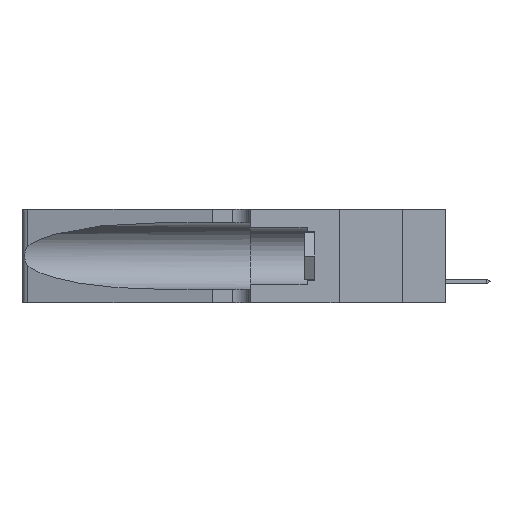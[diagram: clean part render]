
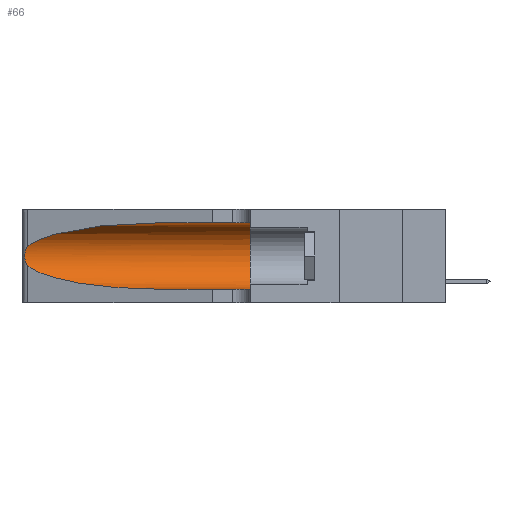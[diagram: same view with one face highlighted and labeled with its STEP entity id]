
A CAD part, left-side view. The second image highlights one B-rep face of the part: STEP entity #66.
In plain terms, the highlighted cylindrical face has radius 3.308 mm (diameter 6.617 mm), a partial arc.
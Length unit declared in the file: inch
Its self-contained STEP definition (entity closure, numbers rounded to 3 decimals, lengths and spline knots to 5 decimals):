
#31 = CARTESIAN_POINT ( 'NONE',  ( 0.25555, 1.22994, 0.2215 ) ) ;
#66 = ADVANCED_FACE ( 'NONE', ( #11929 ), #21941, .F. ) ;
#129 = CARTESIAN_POINT ( 'NONE',  ( 0.2373, 1.15595, 0.28018 ) ) ;
#564 = CARTESIAN_POINT ( 'NONE',  ( 0.1305, 1.61858, 0.185 ) ) ;
#613 = ORIENTED_EDGE ( 'NONE', *, *, #24819, .T. ) ;
#1455 = VECTOR ( 'NONE', #21674, 39.37008 ) ;
#1621 = CARTESIAN_POINT ( 'NONE',  ( 0.25487, 1.22718, 0.14631 ) ) ;
#1700 = DIRECTION ( 'NONE',  ( 0., -1., 0. ) ) ;
#2031 = CARTESIAN_POINT ( 'NONE',  ( 0.25854, 1.2359, 0.20912 ) ) ;
#2060 = CARTESIAN_POINT ( 'NONE',  ( 0.18966, 0.96281, 0.31525 ) ) ;
#2121 = CIRCLE ( 'NONE', #2486, 0.13025 ) ;
#2486 = AXIS2_PLACEMENT_3D ( 'NONE', #12428, #10633, #6418 ) ;
#3036 = VERTEX_POINT ( 'NONE', #6932 ) ;
#4515 = ORIENTED_EDGE ( 'NONE', *, *, #13073, .T. ) ;
#5022 = ORIENTED_EDGE ( 'NONE', *, *, #16414, .T. ) ;
#5615 = CARTESIAN_POINT ( 'NONE',  ( 0.1305, 1.61858, 0.31525 ) ) ;
#5694 = CARTESIAN_POINT ( 'NONE',  ( 0.1305, 0.72297, 0.05475 ) ) ;
#5758 = EDGE_CURVE ( 'NONE', #8298, #3036, #2121, .T. ) ;
#5880 = CARTESIAN_POINT ( 'NONE',  ( 0.26018, 1.23835, 0.19895 ) ) ;
#5958 = CARTESIAN_POINT ( 'NONE',  ( 0.25555, 1.22993, 0.14849 ) ) ;
#6418 = DIRECTION ( 'NONE',  ( 0., 0., 1. ) ) ;
#6715 = VECTOR ( 'NONE', #1700, 39.37008 ) ;
#6932 = CARTESIAN_POINT ( 'NONE',  ( 0.1305, 0.35, 0.05475 ) ) ;
#7156 = EDGE_CURVE ( 'NONE', #19594, #8298, #17470, .T. ) ;
#7443 = CARTESIAN_POINT ( 'NONE',  ( 0.2373, 1.15595, 0.08982 ) ) ;
#7899 = CARTESIAN_POINT ( 'NONE',  ( 0.25856, 1.23593, 0.16098 ) ) ;
#8298 = VERTEX_POINT ( 'NONE', #21575 ) ;
#8544 =( BOUNDED_CURVE ( )  B_SPLINE_CURVE ( 3, ( #9401, #7443, #11524, #5694 ),
 .UNSPECIFIED., .F., .F. ) 
 B_SPLINE_CURVE_WITH_KNOTS ( ( 4, 4 ),
 ( 3.44316, 4.71239 ),
 .UNSPECIFIED. ) 
 CURVE ( )  GEOMETRIC_REPRESENTATION_ITEM ( )  RATIONAL_B_SPLINE_CURVE ( ( 1., 0.87, 0.87, 1. ) ) 
 REPRESENTATION_ITEM ( '' )  );
#8830 = ORIENTED_EDGE ( 'NONE', *, *, #7156, .F. ) ;
#9401 = CARTESIAN_POINT ( 'NONE',  ( 0.25487, 1.22718, 0.14631 ) ) ;
#9952 = LINE ( 'NONE', #13614, #1455 ) ;
#10029 = CARTESIAN_POINT ( 'NONE',  ( 0.26075, 1.23896, 0.19203 ) ) ;
#10633 = DIRECTION ( 'NONE',  ( 0., 1., 0. ) ) ;
#10772 = DIRECTION ( 'NONE',  ( 0., -1., 0. ) ) ;
#11154 = VERTEX_POINT ( 'NONE', #1621 ) ;
#11524 = CARTESIAN_POINT ( 'NONE',  ( 0.18966, 0.96281, 0.05475 ) ) ;
#11929 = FACE_OUTER_BOUND ( 'NONE', #17820, .T. ) ;
#12145 = CARTESIAN_POINT ( 'NONE',  ( 0.25639, 1.23184, 0.21858 ) ) ;
#12428 = CARTESIAN_POINT ( 'NONE',  ( 0.1305, 0.35, 0.185 ) ) ;
#12782 = DIRECTION ( 'NONE',  ( 0., 0., -1. ) ) ;
#13073 = EDGE_CURVE ( 'NONE', #15684, #3036, #9952, .T. ) ;
#13614 = CARTESIAN_POINT ( 'NONE',  ( 0.1305, 1.61858, 0.05475 ) ) ;
#14082 = CARTESIAN_POINT ( 'NONE',  ( 0.25487, 1.22718, 0.22369 ) ) ;
#14096 = CARTESIAN_POINT ( 'NONE',  ( 0.25787, 1.23484, 0.2124 ) ) ;
#15684 = VERTEX_POINT ( 'NONE', #25708 ) ;
#16414 = EDGE_CURVE ( 'NONE', #11154, #15684, #8544, .T. ) ;
#17204 = EDGE_CURVE ( 'NONE', #22772, #11154, #17460, .T. ) ;
#17460 = B_SPLINE_CURVE_WITH_KNOTS ( 'NONE', 3,
 ( #23967, #31, #12145, #14096, #2031, #5880, #10029, #22051, #24044, #7899, #21971, #18116, #5958, #20030 ),
 .UNSPECIFIED., .F., .F.,
 ( 4, 2, 2, 2, 2, 2, 4 ),
 ( 0., 0.00027, 0.00053, 0.00107, 0.0016, 0.00187, 0.00214 ),
 .UNSPECIFIED. ) ;
#17470 = LINE ( 'NONE', #5615, #6715 ) ;
#17820 = EDGE_LOOP ( 'NONE', ( #613, #21364, #5022, #4515, #20203, #8830 ) ) ;
#18116 = CARTESIAN_POINT ( 'NONE',  ( 0.25639, 1.23186, 0.15144 ) ) ;
#19594 = VERTEX_POINT ( 'NONE', #22977 ) ;
#20030 = CARTESIAN_POINT ( 'NONE',  ( 0.25487, 1.22718, 0.14631 ) ) ;
#20170 =( BOUNDED_CURVE ( )  B_SPLINE_CURVE ( 3, ( #20385, #2060, #129, #22305 ),
 .UNSPECIFIED., .F., .F. ) 
 B_SPLINE_CURVE_WITH_KNOTS ( ( 4, 4 ),
 ( 1.5708, 2.84003 ),
 .UNSPECIFIED. ) 
 CURVE ( )  GEOMETRIC_REPRESENTATION_ITEM ( )  RATIONAL_B_SPLINE_CURVE ( ( 1., 0.87, 0.87, 1. ) ) 
 REPRESENTATION_ITEM ( '' )  );
#20203 = ORIENTED_EDGE ( 'NONE', *, *, #5758, .F. ) ;
#20385 = CARTESIAN_POINT ( 'NONE',  ( 0.1305, 0.72297, 0.31525 ) ) ;
#21202 = AXIS2_PLACEMENT_3D ( 'NONE', #564, #10772, #12782 ) ;
#21364 = ORIENTED_EDGE ( 'NONE', *, *, #17204, .T. ) ;
#21575 = CARTESIAN_POINT ( 'NONE',  ( 0.1305, 0.35, 0.31525 ) ) ;
#21674 = DIRECTION ( 'NONE',  ( 0., -1., 0. ) ) ;
#21941 = CYLINDRICAL_SURFACE ( 'NONE', #21202, 0.13025 ) ;
#21971 = CARTESIAN_POINT ( 'NONE',  ( 0.25789, 1.23486, 0.15765 ) ) ;
#22051 = CARTESIAN_POINT ( 'NONE',  ( 0.26075, 1.23896, 0.178 ) ) ;
#22305 = CARTESIAN_POINT ( 'NONE',  ( 0.25487, 1.22718, 0.22369 ) ) ;
#22772 = VERTEX_POINT ( 'NONE', #14082 ) ;
#22977 = CARTESIAN_POINT ( 'NONE',  ( 0.1305, 0.72297, 0.31525 ) ) ;
#23967 = CARTESIAN_POINT ( 'NONE',  ( 0.25487, 1.22718, 0.22369 ) ) ;
#24044 = CARTESIAN_POINT ( 'NONE',  ( 0.26017, 1.23833, 0.17102 ) ) ;
#24819 = EDGE_CURVE ( 'NONE', #19594, #22772, #20170, .T. ) ;
#25708 = CARTESIAN_POINT ( 'NONE',  ( 0.1305, 0.72297, 0.05475 ) ) ;
